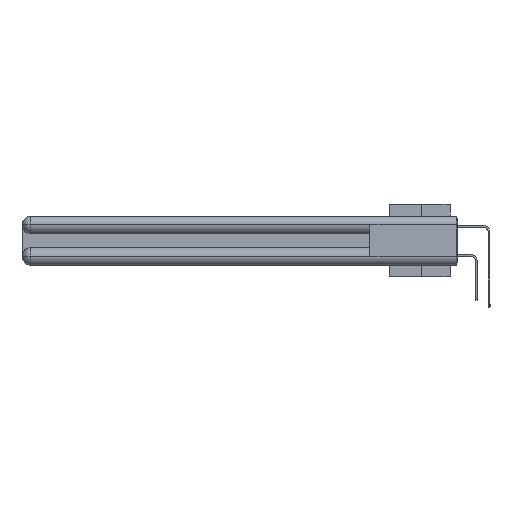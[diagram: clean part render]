
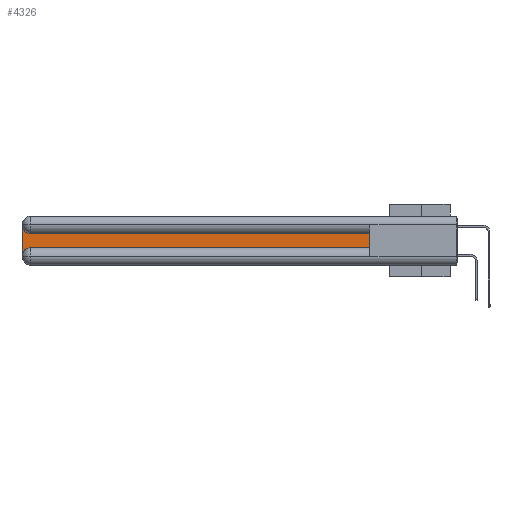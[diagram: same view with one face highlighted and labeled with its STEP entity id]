
A CAD part, left-side view. The second image highlights one B-rep face of the part: STEP entity #4326.
In plain terms, the highlighted planar face has unit normal (-1, 0, 0).
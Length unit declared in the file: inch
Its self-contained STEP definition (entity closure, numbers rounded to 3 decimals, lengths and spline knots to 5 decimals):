
#742 = CIRCLE ( 'NONE', #9310, 0.06 ) ;
#1429 = LINE ( 'NONE', #31770, #20200 ) ;
#2544 = CARTESIAN_POINT ( 'NONE',  ( 0.075, 2.94, -0.0625 ) ) ;
#4326 = ADVANCED_FACE ( 'NONE', ( #24076 ), #7634, .F. ) ;
#4697 = VERTEX_POINT ( 'NONE', #13286 ) ;
#5472 = AXIS2_PLACEMENT_3D ( 'NONE', #19050, #18348, #18865 ) ;
#5654 = DIRECTION ( 'NONE',  ( 0., 0., -1. ) ) ;
#5974 = CARTESIAN_POINT ( 'NONE',  ( 0.075, 3., -0.2775 ) ) ;
#6771 = VERTEX_POINT ( 'NONE', #28411 ) ;
#7634 = PLANE ( 'NONE',  #5472 ) ;
#9310 = AXIS2_PLACEMENT_3D ( 'NONE', #19036, #13139, #5654 ) ;
#9813 = DIRECTION ( 'NONE',  ( 0., 0., 1. ) ) ;
#10094 = VERTEX_POINT ( 'NONE', #18009 ) ;
#10323 = EDGE_CURVE ( 'NONE', #10094, #16002, #21955, .T. ) ;
#10451 = EDGE_LOOP ( 'NONE', ( #32431, #34373, #33330, #16877, #19999, #19127 ) ) ;
#11612 = VERTEX_POINT ( 'NONE', #26984 ) ;
#11706 = AXIS2_PLACEMENT_3D ( 'NONE', #2544, #24524, #27718 ) ;
#12069 = CARTESIAN_POINT ( 'NONE',  ( 0.075, 0.6, -0.2175 ) ) ;
#12241 = CIRCLE ( 'NONE', #11706, 0.06 ) ;
#13139 = DIRECTION ( 'NONE',  ( 1., 0., 0. ) ) ;
#13278 = DIRECTION ( 'NONE',  ( 0., 1., 0. ) ) ;
#13286 = CARTESIAN_POINT ( 'NONE',  ( 0.075, 0.6, -0.1225 ) ) ;
#13316 = EDGE_CURVE ( 'NONE', #11612, #34355, #22542, .T. ) ;
#15360 = EDGE_CURVE ( 'NONE', #16002, #11612, #742, .T. ) ;
#16002 = VERTEX_POINT ( 'NONE', #5974 ) ;
#16130 = LINE ( 'NONE', #34924, #25470 ) ;
#16877 = ORIENTED_EDGE ( 'NONE', *, *, #15360, .T. ) ;
#18009 = CARTESIAN_POINT ( 'NONE',  ( 0.075, 3., -0.0625 ) ) ;
#18348 = DIRECTION ( 'NONE',  ( 1., 0., 0. ) ) ;
#18704 = DIRECTION ( 'NONE',  ( 0., 0., -1. ) ) ;
#18861 = EDGE_CURVE ( 'NONE', #6771, #10094, #12241, .T. ) ;
#18865 = DIRECTION ( 'NONE',  ( 0., 0., -1. ) ) ;
#19036 = CARTESIAN_POINT ( 'NONE',  ( 0.075, 2.94, -0.2775 ) ) ;
#19050 = CARTESIAN_POINT ( 'NONE',  ( 0.075, 3., -0.1225 ) ) ;
#19127 = ORIENTED_EDGE ( 'NONE', *, *, #31454, .T. ) ;
#19252 = CARTESIAN_POINT ( 'NONE',  ( 0.075, 3., -0.2175 ) ) ;
#19999 = ORIENTED_EDGE ( 'NONE', *, *, #13316, .T. ) ;
#20200 = VECTOR ( 'NONE', #9813, 39.37008 ) ;
#21955 = LINE ( 'NONE', #19252, #28395 ) ;
#22542 = LINE ( 'NONE', #25024, #27433 ) ;
#22716 = DIRECTION ( 'NONE',  ( 0., -1., 0. ) ) ;
#24076 = FACE_OUTER_BOUND ( 'NONE', #10451, .T. ) ;
#24524 = DIRECTION ( 'NONE',  ( 1., 0., 0. ) ) ;
#25024 = CARTESIAN_POINT ( 'NONE',  ( 0.075, 0.6, -0.2175 ) ) ;
#25470 = VECTOR ( 'NONE', #13278, 39.37008 ) ;
#26984 = CARTESIAN_POINT ( 'NONE',  ( 0.075, 2.94, -0.2175 ) ) ;
#27433 = VECTOR ( 'NONE', #22716, 39.37008 ) ;
#27718 = DIRECTION ( 'NONE',  ( 0., 0., -1. ) ) ;
#28395 = VECTOR ( 'NONE', #18704, 39.37008 ) ;
#28411 = CARTESIAN_POINT ( 'NONE',  ( 0.075, 2.94, -0.1225 ) ) ;
#31454 = EDGE_CURVE ( 'NONE', #34355, #4697, #1429, .T. ) ;
#31770 = CARTESIAN_POINT ( 'NONE',  ( 0.075, 0.6, -0.2175 ) ) ;
#32431 = ORIENTED_EDGE ( 'NONE', *, *, #34463, .T. ) ;
#33330 = ORIENTED_EDGE ( 'NONE', *, *, #10323, .T. ) ;
#34355 = VERTEX_POINT ( 'NONE', #12069 ) ;
#34373 = ORIENTED_EDGE ( 'NONE', *, *, #18861, .T. ) ;
#34463 = EDGE_CURVE ( 'NONE', #4697, #6771, #16130, .T. ) ;
#34924 = CARTESIAN_POINT ( 'NONE',  ( 0.075, 0.6, -0.1225 ) ) ;
